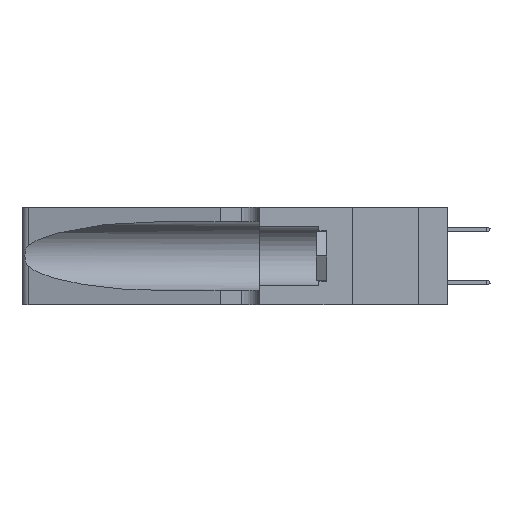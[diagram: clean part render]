
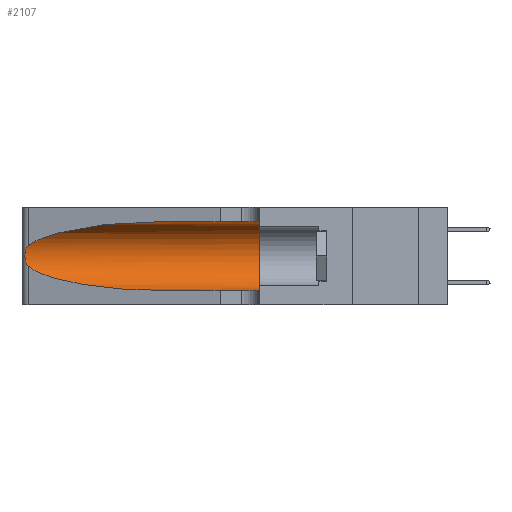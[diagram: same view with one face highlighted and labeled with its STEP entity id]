
A CAD part, left-side view. The second image highlights one B-rep face of the part: STEP entity #2107.
In plain terms, the highlighted cylindrical face has radius 3.308 mm (diameter 6.617 mm), a partial arc.
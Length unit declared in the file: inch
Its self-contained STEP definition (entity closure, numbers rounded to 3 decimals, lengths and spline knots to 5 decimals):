
#402 = VERTEX_POINT ( 'NONE', #34169 ) ;
#813 = EDGE_CURVE ( 'NONE', #46850, #5840, #24964, .T. ) ;
#2107 = ADVANCED_FACE ( 'NONE', ( #38164 ), #46426, .F. ) ;
#2553 = CARTESIAN_POINT ( 'NONE',  ( 0.25487, 1.22718, 0.14631 ) ) ;
#4252 = CARTESIAN_POINT ( 'NONE',  ( 0.2373, 1.15595, 0.08982 ) ) ;
#5164 = EDGE_LOOP ( 'NONE', ( #20022, #13140, #31865, #26109, #12704, #12330 ) ) ;
#5791 = DIRECTION ( 'NONE',  ( 0., -1., 0. ) ) ;
#5840 = VERTEX_POINT ( 'NONE', #18477 ) ;
#6236 = CARTESIAN_POINT ( 'NONE',  ( 0.25639, 1.23184, 0.21858 ) ) ;
#7092 =( BOUNDED_CURVE ( )  B_SPLINE_CURVE ( 3, ( #30485, #4252, #11898, #37920 ),
 .UNSPECIFIED., .F., .F. ) 
 B_SPLINE_CURVE_WITH_KNOTS ( ( 4, 4 ),
 ( 3.44316, 4.71239 ),
 .UNSPECIFIED. ) 
 CURVE ( )  GEOMETRIC_REPRESENTATION_ITEM ( )  RATIONAL_B_SPLINE_CURVE ( ( 1., 0.87, 0.87, 1. ) ) 
 REPRESENTATION_ITEM ( '' )  );
#8462 = DIRECTION ( 'NONE',  ( 0., 1., 0. ) ) ;
#8838 = VERTEX_POINT ( 'NONE', #30605 ) ;
#10071 = CARTESIAN_POINT ( 'NONE',  ( 0.25854, 1.2359, 0.20912 ) ) ;
#10485 = CIRCLE ( 'NONE', #24105, 0.13025 ) ;
#11359 =( BOUNDED_CURVE ( )  B_SPLINE_CURVE ( 3, ( #28846, #32569, #14014, #40011 ),
 .UNSPECIFIED., .F., .T. ) 
 B_SPLINE_CURVE_WITH_KNOTS ( ( 4, 4 ),
 ( 1.5708, 2.84003 ),
 .UNSPECIFIED. ) 
 CURVE ( )  GEOMETRIC_REPRESENTATION_ITEM ( )  RATIONAL_B_SPLINE_CURVE ( ( 1., 0.87, 0.87, 1. ) ) 
 REPRESENTATION_ITEM ( '' )  );
#11898 = CARTESIAN_POINT ( 'NONE',  ( 0.18966, 0.96281, 0.05475 ) ) ;
#12262 = VERTEX_POINT ( 'NONE', #33056 ) ;
#12330 = ORIENTED_EDGE ( 'NONE', *, *, #19465, .F. ) ;
#12704 = ORIENTED_EDGE ( 'NONE', *, *, #19377, .F. ) ;
#13140 = ORIENTED_EDGE ( 'NONE', *, *, #20167, .T. ) ;
#13435 = CARTESIAN_POINT ( 'NONE',  ( 0.1305, 0.72297, 0.05475 ) ) ;
#13803 = CARTESIAN_POINT ( 'NONE',  ( 0.26075, 1.23896, 0.19203 ) ) ;
#14014 = CARTESIAN_POINT ( 'NONE',  ( 0.2373, 1.15595, 0.28018 ) ) ;
#16859 = EDGE_CURVE ( 'NONE', #12262, #8838, #11359, .T. ) ;
#17597 = CARTESIAN_POINT ( 'NONE',  ( 0.26017, 1.23833, 0.17102 ) ) ;
#17884 = CARTESIAN_POINT ( 'NONE',  ( 0.1305, 1.61858, 0.05475 ) ) ;
#18477 = CARTESIAN_POINT ( 'NONE',  ( 0.1305, 0.35, 0.05475 ) ) ;
#19377 = EDGE_CURVE ( 'NONE', #43710, #5840, #10485, .T. ) ;
#19465 = EDGE_CURVE ( 'NONE', #12262, #43710, #25686, .T. ) ;
#19877 = EDGE_CURVE ( 'NONE', #402, #46850, #7092, .T. ) ;
#20022 = ORIENTED_EDGE ( 'NONE', *, *, #16859, .T. ) ;
#20167 = EDGE_CURVE ( 'NONE', #8838, #402, #44611, .T. ) ;
#21354 = CARTESIAN_POINT ( 'NONE',  ( 0.25789, 1.23486, 0.15765 ) ) ;
#23809 = CARTESIAN_POINT ( 'NONE',  ( 0.1305, 0.35, 0.31525 ) ) ;
#24105 = AXIS2_PLACEMENT_3D ( 'NONE', #30843, #8462, #34575 ) ;
#24507 = VECTOR ( 'NONE', #5791, 39.37008 ) ;
#24936 = CARTESIAN_POINT ( 'NONE',  ( 0.25487, 1.22718, 0.22369 ) ) ;
#24964 = LINE ( 'NONE', #17884, #45753 ) ;
#25095 = CARTESIAN_POINT ( 'NONE',  ( 0.25555, 1.22993, 0.14849 ) ) ;
#25686 = LINE ( 'NONE', #39401, #24507 ) ;
#26109 = ORIENTED_EDGE ( 'NONE', *, *, #813, .T. ) ;
#28342 = DIRECTION ( 'NONE',  ( 0., 0., -1. ) ) ;
#28846 = CARTESIAN_POINT ( 'NONE',  ( 0.1305, 0.72297, 0.31525 ) ) ;
#28935 = AXIS2_PLACEMENT_3D ( 'NONE', #35802, #43200, #28342 ) ;
#30485 = CARTESIAN_POINT ( 'NONE',  ( 0.25487, 1.22718, 0.14631 ) ) ;
#30605 = CARTESIAN_POINT ( 'NONE',  ( 0.25487, 1.22718, 0.22369 ) ) ;
#30843 = CARTESIAN_POINT ( 'NONE',  ( 0.1305, 0.35, 0.185 ) ) ;
#31865 = ORIENTED_EDGE ( 'NONE', *, *, #19877, .T. ) ;
#32384 = CARTESIAN_POINT ( 'NONE',  ( 0.25787, 1.23484, 0.2124 ) ) ;
#32569 = CARTESIAN_POINT ( 'NONE',  ( 0.18966, 0.96281, 0.31525 ) ) ;
#33056 = CARTESIAN_POINT ( 'NONE',  ( 0.1305, 0.72297, 0.31525 ) ) ;
#34169 = CARTESIAN_POINT ( 'NONE',  ( 0.25487, 1.22718, 0.14631 ) ) ;
#34575 = DIRECTION ( 'NONE',  ( 0., 0., 1. ) ) ;
#35802 = CARTESIAN_POINT ( 'NONE',  ( 0.1305, 1.61858, 0.185 ) ) ;
#36117 = CARTESIAN_POINT ( 'NONE',  ( 0.26018, 1.23835, 0.19895 ) ) ;
#37920 = CARTESIAN_POINT ( 'NONE',  ( 0.1305, 0.72297, 0.05475 ) ) ;
#38164 = FACE_OUTER_BOUND ( 'NONE', #5164, .T. ) ;
#39401 = CARTESIAN_POINT ( 'NONE',  ( 0.1305, 1.61858, 0.31525 ) ) ;
#39820 = CARTESIAN_POINT ( 'NONE',  ( 0.26075, 1.23896, 0.178 ) ) ;
#40011 = CARTESIAN_POINT ( 'NONE',  ( 0.25487, 1.22718, 0.22369 ) ) ;
#43200 = DIRECTION ( 'NONE',  ( 0., -1., 0. ) ) ;
#43530 = CARTESIAN_POINT ( 'NONE',  ( 0.25856, 1.23593, 0.16098 ) ) ;
#43710 = VERTEX_POINT ( 'NONE', #23809 ) ;
#43805 = DIRECTION ( 'NONE',  ( 0., -1., 0. ) ) ;
#44611 = B_SPLINE_CURVE_WITH_KNOTS ( 'NONE', 3,
 ( #24936, #47023, #6236, #32384, #10071, #36117, #13803, #39820, #17597, #43530, #21354, #47185, #25095, #2553 ),
 .UNSPECIFIED., .F., .F.,
 ( 4, 2, 2, 2, 2, 2, 4 ),
 ( 0., 0.00027, 0.00053, 0.00107, 0.0016, 0.00187, 0.00214 ),
 .UNSPECIFIED. ) ;
#45753 = VECTOR ( 'NONE', #43805, 39.37008 ) ;
#46426 = CYLINDRICAL_SURFACE ( 'NONE', #28935, 0.13025 ) ;
#46850 = VERTEX_POINT ( 'NONE', #13435 ) ;
#47023 = CARTESIAN_POINT ( 'NONE',  ( 0.25555, 1.22994, 0.2215 ) ) ;
#47185 = CARTESIAN_POINT ( 'NONE',  ( 0.25639, 1.23186, 0.15144 ) ) ;
